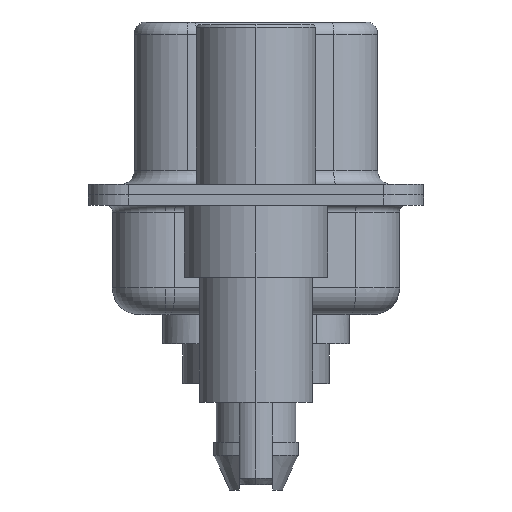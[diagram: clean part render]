
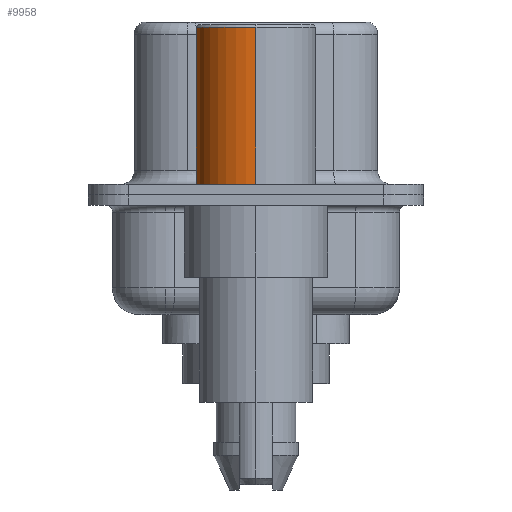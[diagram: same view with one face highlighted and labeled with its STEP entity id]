
A CAD part, left-side view. The second image highlights one B-rep face of the part: STEP entity #9958.
In plain terms, the highlighted cylindrical face has radius 2.25 mm (diameter 4.5 mm), a partial arc.
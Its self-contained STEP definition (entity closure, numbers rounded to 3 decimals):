
#35 = ORIENTED_EDGE ( 'NONE', *, *, #2443, .T. ) ;
#95 = VERTEX_POINT ( 'NONE', #734 ) ;
#448 = AXIS2_PLACEMENT_3D ( 'NONE', #10312, #3041, #11451 ) ;
#734 = CARTESIAN_POINT ( 'NONE',  ( 2.25, 0., 0.4 ) ) ;
#1270 = CARTESIAN_POINT ( 'NONE',  ( 2.25, 0., 6.3 ) ) ;
#1950 = DIRECTION ( 'NONE',  ( 0., 0., 1. ) ) ;
#2443 = EDGE_CURVE ( 'NONE', #4558, #10960, #6235, .T. ) ;
#2968 = DIRECTION ( 'NONE',  ( 1., 0., 0. ) ) ;
#2977 = ORIENTED_EDGE ( 'NONE', *, *, #13308, .F. ) ;
#3041 = DIRECTION ( 'NONE',  ( 0., 0., 1. ) ) ;
#4126 = CARTESIAN_POINT ( 'NONE',  ( 0., 0., 0.581 ) ) ;
#4558 = VERTEX_POINT ( 'NONE', #9889 ) ;
#5135 = CARTESIAN_POINT ( 'NONE',  ( 0., 0., 6.3 ) ) ;
#5850 = VECTOR ( 'NONE', #1950, 1000. ) ;
#5867 = VERTEX_POINT ( 'NONE', #1270 ) ;
#6235 = LINE ( 'NONE', #9486, #5850 ) ;
#6350 = DIRECTION ( 'NONE',  ( 1., 0., 0. ) ) ;
#6825 = CIRCLE ( 'NONE', #12352, 2.25 ) ;
#7271 = CARTESIAN_POINT ( 'NONE',  ( 2.25, 0., 0.581 ) ) ;
#7598 = LINE ( 'NONE', #7271, #8372 ) ;
#7783 = CYLINDRICAL_SURFACE ( 'NONE', #13728, 2.25 ) ;
#8086 = ORIENTED_EDGE ( 'NONE', *, *, #10969, .T. ) ;
#8143 = EDGE_LOOP ( 'NONE', ( #8086, #35, #2977, #15763 ) ) ;
#8170 = FACE_OUTER_BOUND ( 'NONE', #8143, .T. ) ;
#8372 = VECTOR ( 'NONE', #10103, 1000. ) ;
#8477 = EDGE_CURVE ( 'NONE', #95, #5867, #7598, .T. ) ;
#9486 = CARTESIAN_POINT ( 'NONE',  ( -2.25, 0., 0.581 ) ) ;
#9889 = CARTESIAN_POINT ( 'NONE',  ( -2.25, 0., 0.4 ) ) ;
#9958 = ADVANCED_FACE ( 'NONE', ( #8170 ), #7783, .T. ) ;
#10103 = DIRECTION ( 'NONE',  ( 0., 0., 1. ) ) ;
#10243 = DIRECTION ( 'NONE',  ( 0., 0., 1. ) ) ;
#10312 = CARTESIAN_POINT ( 'NONE',  ( 0., 0., 0.4 ) ) ;
#10960 = VERTEX_POINT ( 'NONE', #15170 ) ;
#10969 = EDGE_CURVE ( 'NONE', #95, #4558, #12165, .T. ) ;
#11451 = DIRECTION ( 'NONE',  ( 1., 0., 0. ) ) ;
#12165 = CIRCLE ( 'NONE', #448, 2.25 ) ;
#12352 = AXIS2_PLACEMENT_3D ( 'NONE', #5135, #13639, #6350 ) ;
#13308 = EDGE_CURVE ( 'NONE', #5867, #10960, #6825, .T. ) ;
#13639 = DIRECTION ( 'NONE',  ( 0., 0., 1. ) ) ;
#13728 = AXIS2_PLACEMENT_3D ( 'NONE', #4126, #10243, #2968 ) ;
#15170 = CARTESIAN_POINT ( 'NONE',  ( -2.25, 0., 6.3 ) ) ;
#15763 = ORIENTED_EDGE ( 'NONE', *, *, #8477, .F. ) ;
